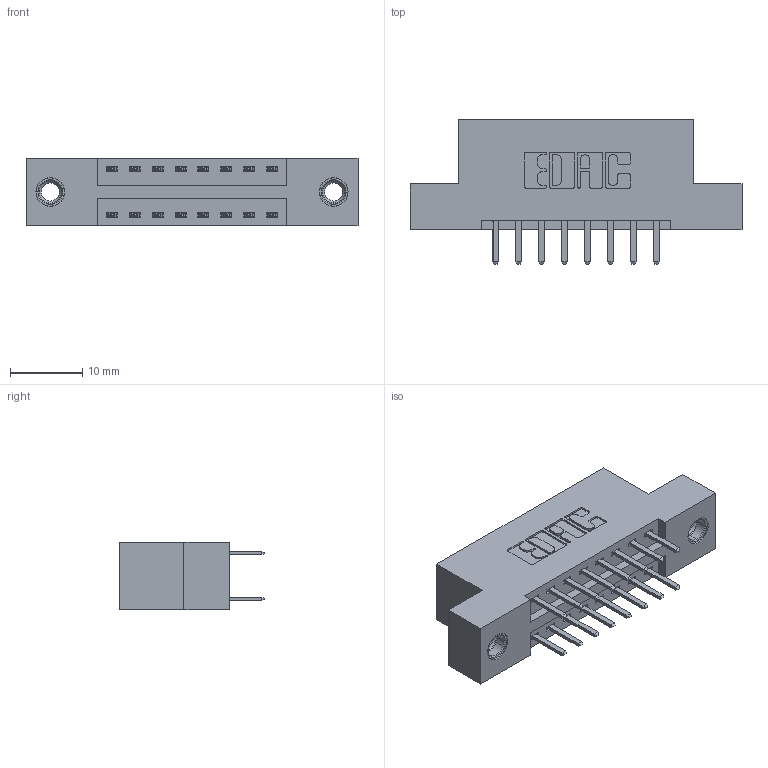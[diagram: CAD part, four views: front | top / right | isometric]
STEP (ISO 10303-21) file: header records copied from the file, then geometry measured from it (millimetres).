
FILE_DESCRIPTION (( 'STEP AP203' ), '1' );
FILE_NAME ('346-016-520-207.STEP', '2022-05-18T15:21:17', ( '' ), ( '' ), 'SwSTEP 2.0', 'SolidWorks 2020', '' );
FILE_SCHEMA (( 'CONFIG_CONTROL_DESIGN' ));
Length unit declared in the file: inch
Products named in the file (4): 345-292-001_345-293-120; 345-250-001_345-250-005-103; 346 Part_Flush Mounting Lugs - 0.156 Dia-TI; 346-016-520-207
Assembly tree (19 placements, depth 2):
  346-016-520-207
    346 Part_Flush Mounting Lugs - 0.156 Dia-TI
    345-292-001_345-293-120  x16
    345-250-001_345-250-005-103  x2
Bounding box: 45.97 x 20.02 x 9.4 mm (x, y, z)
Volume: 4198.4 mm3; surface area: 5253.9 mm2
Topology: 19 solids, 19 shells, 1078 faces, 3073 edges, 1998 vertices
Faces by surface type: plane 700, cylinder 362, cone 12, torus 4
Entity records: 11098 total; most frequent: CARTESIAN_POINT 1871, ORIENTED_EDGE 1786, DIRECTION 1715, EDGE_CURVE 893, LINE 705, VECTOR 705, VERTEX_POINT 588, AXIS2_PLACEMENT_3D 505
